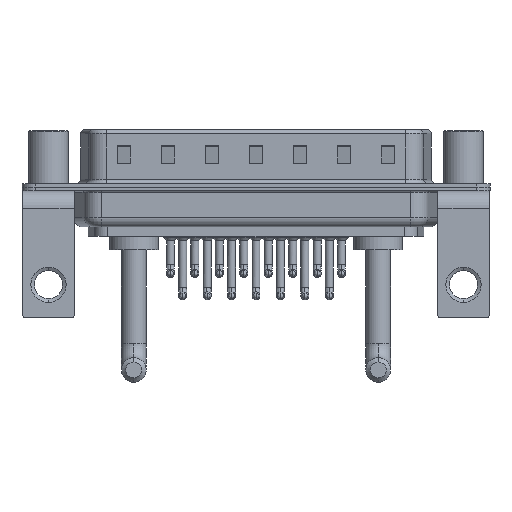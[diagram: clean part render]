
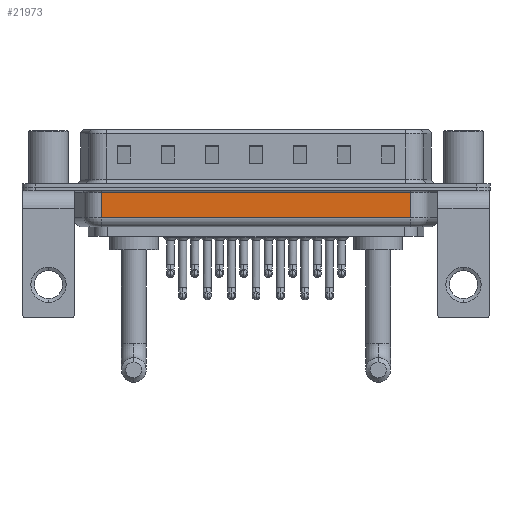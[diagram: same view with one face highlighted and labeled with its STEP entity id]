
A CAD part, front view. The second image highlights one B-rep face of the part: STEP entity #21973.
In plain terms, the highlighted planar face has unit normal (0, -1, 0).
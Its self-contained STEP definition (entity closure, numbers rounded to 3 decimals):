
#1293 = ORIENTED_EDGE ( 'NONE', *, *, #7062, .T. ) ;
#1932 = AXIS2_PLACEMENT_3D ( 'NONE', #6674, #23461, #13014 ) ;
#2207 = VECTOR ( 'NONE', #24069, 1000. ) ;
#3067 = ORIENTED_EDGE ( 'NONE', *, *, #16710, .F. ) ;
#5307 = VERTEX_POINT ( 'NONE', #9584 ) ;
#6243 = ORIENTED_EDGE ( 'NONE', *, *, #19841, .T. ) ;
#6414 = VECTOR ( 'NONE', #15615, 1000. ) ;
#6586 = DIRECTION ( 'NONE',  ( -1., 0., 0. ) ) ;
#6674 = CARTESIAN_POINT ( 'NONE',  ( 6.006, -5.35, -4.5 ) ) ;
#7062 = EDGE_CURVE ( 'NONE', #20334, #5307, #20175, .T. ) ;
#7276 = DIRECTION ( 'NONE',  ( 1., 0., 0. ) ) ;
#8352 = VECTOR ( 'NONE', #6586, 1000. ) ;
#9334 = VECTOR ( 'NONE', #7276, 1000. ) ;
#9584 = CARTESIAN_POINT ( 'NONE',  ( 41.044, -5.35, -0.65 ) ) ;
#9882 = LINE ( 'NONE', #15947, #2207 ) ;
#10970 = VERTEX_POINT ( 'NONE', #11621 ) ;
#11287 = ORIENTED_EDGE ( 'NONE', *, *, #12207, .T. ) ;
#11621 = CARTESIAN_POINT ( 'NONE',  ( 6.006, -5.35, -3.5 ) ) ;
#11876 = FACE_OUTER_BOUND ( 'NONE', #11919, .T. ) ;
#11919 = EDGE_LOOP ( 'NONE', ( #3067, #6243, #1293, #11287 ) ) ;
#12207 = EDGE_CURVE ( 'NONE', #5307, #18490, #17059, .T. ) ;
#13014 = DIRECTION ( 'NONE',  ( 0., 0., 1. ) ) ;
#13968 = CARTESIAN_POINT ( 'NONE',  ( 41.044, -5.35, -4.5 ) ) ;
#15615 = DIRECTION ( 'NONE',  ( 0., 0., 1. ) ) ;
#15947 = CARTESIAN_POINT ( 'NONE',  ( 6.006, -5.35, -4.5 ) ) ;
#16710 = EDGE_CURVE ( 'NONE', #10970, #18490, #9882, .T. ) ;
#17059 = LINE ( 'NONE', #25437, #8352 ) ;
#17739 = CARTESIAN_POINT ( 'NONE',  ( 6.006, -5.35, -3.5 ) ) ;
#18490 = VERTEX_POINT ( 'NONE', #23766 ) ;
#19841 = EDGE_CURVE ( 'NONE', #10970, #20334, #24073, .T. ) ;
#20175 = LINE ( 'NONE', #13968, #6414 ) ;
#20281 = PLANE ( 'NONE',  #1932 ) ;
#20334 = VERTEX_POINT ( 'NONE', #22489 ) ;
#21973 = ADVANCED_FACE ( 'NONE', ( #11876 ), #20281, .F. ) ;
#22489 = CARTESIAN_POINT ( 'NONE',  ( 41.044, -5.35, -3.5 ) ) ;
#23461 = DIRECTION ( 'NONE',  ( 0., 1., 0. ) ) ;
#23766 = CARTESIAN_POINT ( 'NONE',  ( 6.006, -5.35, -0.65 ) ) ;
#24069 = DIRECTION ( 'NONE',  ( 0., 0., 1. ) ) ;
#24073 = LINE ( 'NONE', #17739, #9334 ) ;
#25437 = CARTESIAN_POINT ( 'NONE',  ( 6.006, -5.35, -0.65 ) ) ;
